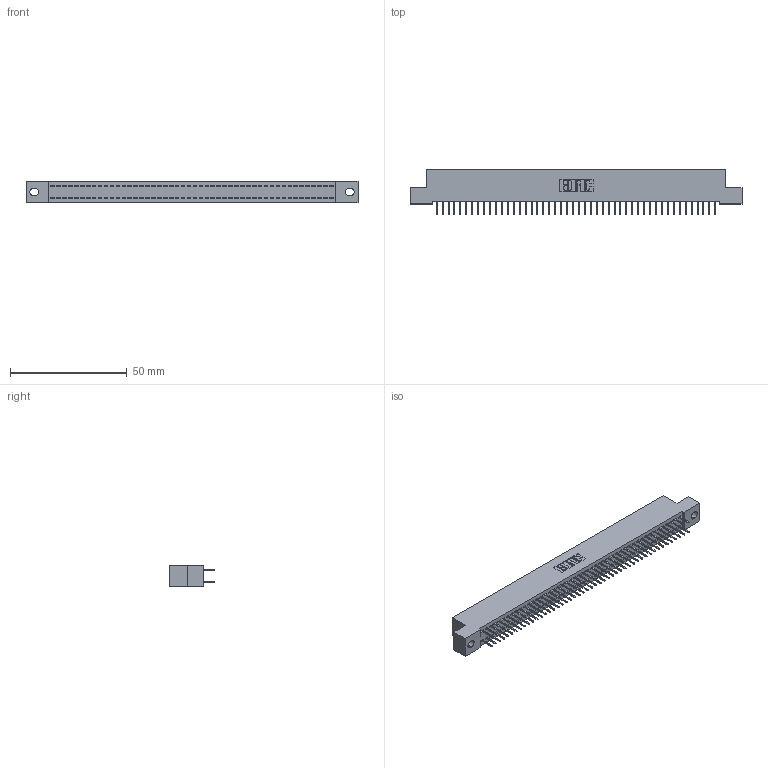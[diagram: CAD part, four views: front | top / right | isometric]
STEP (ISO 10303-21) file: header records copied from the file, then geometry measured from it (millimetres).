
FILE_DESCRIPTION (( 'STEP AP203' ), '1' );
FILE_NAME ('342-096-524-202.STEP', '2019-10-04T15:59:57', ( '' ), ( '' ), 'SwSTEP 2.0', 'SolidWorks 2016', '' );
FILE_SCHEMA (( 'CONFIG_CONTROL_DESIGN' ));
Length unit declared in the file: inch
Products named in the file (3): 345-292-001_345-293-124; 342-096-524-202; 342 Part_.128 Slot
Assembly tree (97 placements, depth 2):
  342-096-524-202
    342 Part_.128 Slot
    345-292-001_345-293-124  x96
Bounding box: 142.24 x 19.69 x 9.4 mm (x, y, z)
Volume: 12611.2 mm3; surface area: 20057.3 mm2
Topology: 97 solids, 97 shells, 5490 faces, 15575 edges, 9998 vertices
Faces by surface type: plane 4102, cylinder 1388
Entity records: 30181 total; most frequent: CARTESIAN_POINT 4994, ORIENTED_EDGE 4930, DIRECTION 4257, EDGE_CURVE 2465, VECTOR 2341, LINE 2341, VERTEX_POINT 1638, AXIS2_PLACEMENT_3D 958
